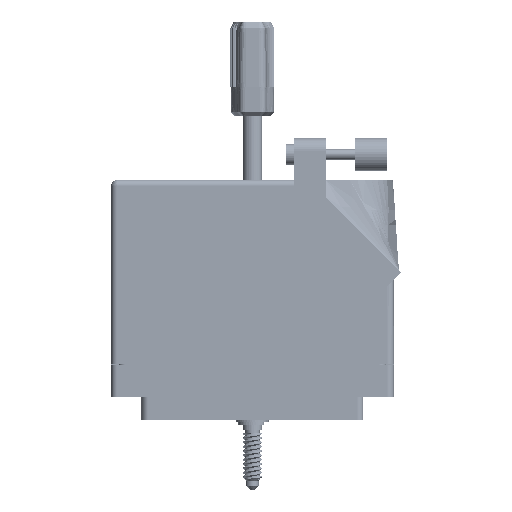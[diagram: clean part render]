
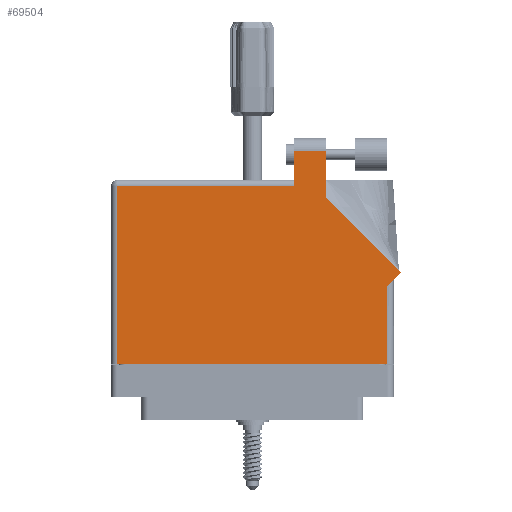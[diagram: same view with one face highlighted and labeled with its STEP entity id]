
A CAD part, front view. The second image highlights one B-rep face of the part: STEP entity #69504.
In plain terms, the highlighted face is planar.
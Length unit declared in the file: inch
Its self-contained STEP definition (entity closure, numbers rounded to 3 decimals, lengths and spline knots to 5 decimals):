
#1019 = DIRECTION ( 'NONE',  ( -0.707, 0.707, 0. ) ) ;
#1785 = CARTESIAN_POINT ( 'NONE',  ( -1.297, 1.613, 0.617 ) ) ;
#1889 = VECTOR ( 'NONE', #33249, 39.37008 ) ;
#3409 = VECTOR ( 'NONE', #62910, 39.37008 ) ;
#5810 = LINE ( 'NONE', #55400, #36310 ) ;
#6772 = DIRECTION ( 'NONE',  ( 0., 1., 0. ) ) ;
#9588 = CARTESIAN_POINT ( 'NONE',  ( 0.706, 1.50942, 0.617 ) ) ;
#9729 = ORIENTED_EDGE ( 'NONE', *, *, #66281, .T. ) ;
#11144 = VECTOR ( 'NONE', #6772, 39.37008 ) ;
#11709 = LINE ( 'NONE', #42222, #3409 ) ;
#13855 = VERTEX_POINT ( 'NONE', #23768 ) ;
#14172 = VERTEX_POINT ( 'NONE', #1785 ) ;
#14890 = EDGE_CURVE ( 'NONE', #18927, #48668, #59836, .T. ) ;
#15326 = DIRECTION ( 'NONE',  ( 0., 0., -1. ) ) ;
#15616 = PLANE ( 'NONE',  #60246 ) ;
#15835 = ORIENTED_EDGE ( 'NONE', *, *, #73879, .T. ) ;
#15887 = CARTESIAN_POINT ( 'NONE',  ( 1.42971, 0.78571, 0.617 ) ) ;
#16656 = CARTESIAN_POINT ( 'NONE',  ( -1.297, -0.1, 0.617 ) ) ;
#17910 = CARTESIAN_POINT ( 'NONE',  ( -1.359, 1.613, 0.617 ) ) ;
#18927 = VERTEX_POINT ( 'NONE', #15887 ) ;
#20790 = LINE ( 'NONE', #9588, #27167 ) ;
#21633 = CARTESIAN_POINT ( 'NONE',  ( 0.399, 1.613, 0.617 ) ) ;
#23130 = DIRECTION ( 'NONE',  ( 0., 1., 0. ) ) ;
#23768 = CARTESIAN_POINT ( 'NONE',  ( 1.297, 0.653, 0.617 ) ) ;
#24107 = VECTOR ( 'NONE', #71208, 39.37008 ) ;
#26260 = EDGE_CURVE ( 'NONE', #13855, #18927, #51519, .T. ) ;
#27056 = LINE ( 'NONE', #62780, #69912 ) ;
#27167 = VECTOR ( 'NONE', #23130, 39.37008 ) ;
#29376 = EDGE_CURVE ( 'NONE', #67826, #13855, #61433, .T. ) ;
#30924 = CARTESIAN_POINT ( 'NONE',  ( 1.359, 0.715, 0.617 ) ) ;
#33249 = DIRECTION ( 'NONE',  ( -1., 0., 0. ) ) ;
#33714 = VECTOR ( 'NONE', #1019, 39.37008 ) ;
#34708 = EDGE_CURVE ( 'NONE', #14172, #48052, #11709, .T. ) ;
#34745 = CARTESIAN_POINT ( 'NONE',  ( -1.359, 1.675, 0.617 ) ) ;
#36310 = VECTOR ( 'NONE', #63506, 39.37008 ) ;
#38997 = VECTOR ( 'NONE', #71230, 39.37008 ) ;
#41772 = LINE ( 'NONE', #45584, #1889 ) ;
#42222 = CARTESIAN_POINT ( 'NONE',  ( -1.297, -0.1, 0.617 ) ) ;
#42802 = ORIENTED_EDGE ( 'NONE', *, *, #34708, .T. ) ;
#45011 = CARTESIAN_POINT ( 'NONE',  ( 0.399, 1.95, 0.617 ) ) ;
#45197 = ORIENTED_EDGE ( 'NONE', *, *, #14890, .T. ) ;
#45584 = CARTESIAN_POINT ( 'NONE',  ( 0.399, 1.95, 0.617 ) ) ;
#45585 = ORIENTED_EDGE ( 'NONE', *, *, #61819, .T. ) ;
#46364 = CARTESIAN_POINT ( 'NONE',  ( 1.297, 0.715, 0.617 ) ) ;
#48052 = VERTEX_POINT ( 'NONE', #16656 ) ;
#48506 = DIRECTION ( 'NONE',  ( -1., 0., 0. ) ) ;
#48668 = VERTEX_POINT ( 'NONE', #73589 ) ;
#50283 = DIRECTION ( 'NONE',  ( 0., -1., 0. ) ) ;
#50630 = EDGE_CURVE ( 'NONE', #48668, #76954, #20790, .T. ) ;
#51519 = LINE ( 'NONE', #30924, #38997 ) ;
#52931 = ORIENTED_EDGE ( 'NONE', *, *, #50630, .T. ) ;
#55400 = CARTESIAN_POINT ( 'NONE',  ( -1.359, -0.1, 0.617 ) ) ;
#56807 = CARTESIAN_POINT ( 'NONE',  ( 0.706, 1.95, 0.617 ) ) ;
#58702 = EDGE_LOOP ( 'NONE', ( #52931, #15835, #45585, #9729, #42802, #79012, #61477, #79862, #45197 ) ) ;
#59836 = LINE ( 'NONE', #61317, #33714 ) ;
#60246 = AXIS2_PLACEMENT_3D ( 'NONE', #34745, #15326, #48506 ) ;
#61317 = CARTESIAN_POINT ( 'NONE',  ( 1.42971, 0.78571, 0.617 ) ) ;
#61433 = LINE ( 'NONE', #46364, #11144 ) ;
#61477 = ORIENTED_EDGE ( 'NONE', *, *, #29376, .T. ) ;
#61819 = EDGE_CURVE ( 'NONE', #73679, #83695, #27056, .T. ) ;
#62780 = CARTESIAN_POINT ( 'NONE',  ( 0.399, 1.675, 0.617 ) ) ;
#62910 = DIRECTION ( 'NONE',  ( 0., -1., 0. ) ) ;
#63506 = DIRECTION ( 'NONE',  ( 1., 0., 0. ) ) ;
#66281 = EDGE_CURVE ( 'NONE', #83695, #14172, #79605, .T. ) ;
#67826 = VERTEX_POINT ( 'NONE', #74763 ) ;
#69504 = ADVANCED_FACE ( 'NONE', ( #74899 ), #15616, .F. ) ;
#69912 = VECTOR ( 'NONE', #50283, 39.37008 ) ;
#71208 = DIRECTION ( 'NONE',  ( -1., 0., 0. ) ) ;
#71230 = DIRECTION ( 'NONE',  ( 0.707, 0.707, 0. ) ) ;
#73589 = CARTESIAN_POINT ( 'NONE',  ( 0.706, 1.50942, 0.617 ) ) ;
#73679 = VERTEX_POINT ( 'NONE', #45011 ) ;
#73879 = EDGE_CURVE ( 'NONE', #76954, #73679, #41772, .T. ) ;
#74763 = CARTESIAN_POINT ( 'NONE',  ( 1.297, -0.1, 0.617 ) ) ;
#74899 = FACE_OUTER_BOUND ( 'NONE', #58702, .T. ) ;
#76954 = VERTEX_POINT ( 'NONE', #56807 ) ;
#77905 = EDGE_CURVE ( 'NONE', #48052, #67826, #5810, .T. ) ;
#79012 = ORIENTED_EDGE ( 'NONE', *, *, #77905, .T. ) ;
#79605 = LINE ( 'NONE', #17910, #24107 ) ;
#79862 = ORIENTED_EDGE ( 'NONE', *, *, #26260, .T. ) ;
#83695 = VERTEX_POINT ( 'NONE', #21633 ) ;
